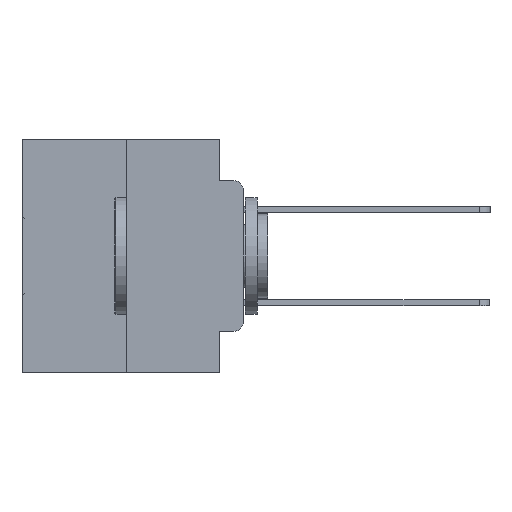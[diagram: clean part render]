
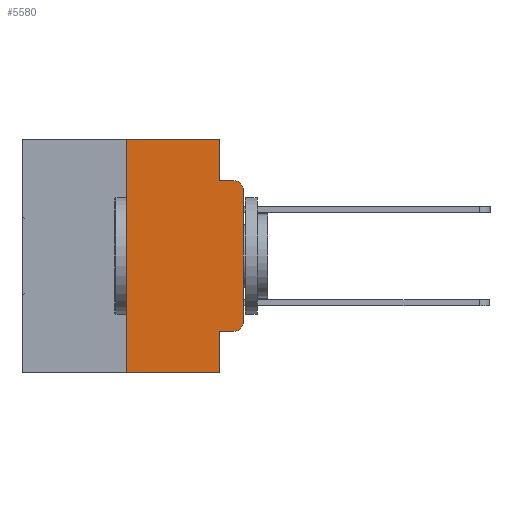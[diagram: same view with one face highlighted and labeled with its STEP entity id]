
A CAD part, left-side view. The second image highlights one B-rep face of the part: STEP entity #5580.
In plain terms, the highlighted planar face has unit normal (-1, 0, 0).
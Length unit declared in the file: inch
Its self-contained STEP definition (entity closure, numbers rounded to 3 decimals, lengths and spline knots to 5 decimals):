
#1508 = VERTEX_POINT ( 'NONE', #18379 ) ;
#1901 = AXIS2_PLACEMENT_3D ( 'NONE', #23226, #7736, #25802 ) ;
#2089 = CARTESIAN_POINT ( 'NONE',  ( 0., 0., -0.3915 ) ) ;
#2698 = CARTESIAN_POINT ( 'NONE',  ( 0., 0.051, 0. ) ) ;
#4531 = VECTOR ( 'NONE', #22962, 39.37008 ) ;
#4701 = EDGE_CURVE ( 'NONE', #5021, #1508, #15655, .T. ) ;
#5004 = AXIS2_PLACEMENT_3D ( 'NONE', #18978, #13904, #31989 ) ;
#5021 = VERTEX_POINT ( 'NONE', #19352 ) ;
#5310 = LINE ( 'NONE', #20338, #4531 ) ;
#5507 = LINE ( 'NONE', #14008, #32211 ) ;
#5580 = ADVANCED_FACE ( 'NONE', ( #9167 ), #13799, .F. ) ;
#6007 = EDGE_CURVE ( 'NONE', #32028, #27870, #29328, .T. ) ;
#6123 = VECTOR ( 'NONE', #23353, 39.37008 ) ;
#7227 = LINE ( 'NONE', #28027, #20176 ) ;
#7736 = DIRECTION ( 'NONE',  ( -1., 0., 0. ) ) ;
#7873 = EDGE_CURVE ( 'NONE', #24982, #12171, #5310, .T. ) ;
#7877 = DIRECTION ( 'NONE',  ( 0., 0., 1. ) ) ;
#8230 = ORIENTED_EDGE ( 'NONE', *, *, #7873, .T. ) ;
#8566 = EDGE_CURVE ( 'NONE', #12171, #15142, #11741, .T. ) ;
#9167 = FACE_OUTER_BOUND ( 'NONE', #31209, .T. ) ;
#9393 = EDGE_CURVE ( 'NONE', #18142, #24982, #27039, .T. ) ;
#10222 = ORIENTED_EDGE ( 'NONE', *, *, #30271, .F. ) ;
#10917 = VECTOR ( 'NONE', #22085, 39.37008 ) ;
#11630 = CARTESIAN_POINT ( 'NONE',  ( 0., 0.051, -0.4115 ) ) ;
#11741 = CIRCLE ( 'NONE', #28651, 0.02 ) ;
#12171 = VERTEX_POINT ( 'NONE', #19094 ) ;
#12544 = ORIENTED_EDGE ( 'NONE', *, *, #25397, .F. ) ;
#12953 = CARTESIAN_POINT ( 'NONE',  ( 0., 0.02, -0.1085 ) ) ;
#13072 = CARTESIAN_POINT ( 'NONE',  ( 0., 0.25, 0. ) ) ;
#13098 = ORIENTED_EDGE ( 'NONE', *, *, #4701, .F. ) ;
#13647 = EDGE_CURVE ( 'NONE', #31257, #23608, #20345, .T. ) ;
#13799 = PLANE ( 'NONE',  #5004 ) ;
#13904 = DIRECTION ( 'NONE',  ( 1., 0., 0. ) ) ;
#13960 = VECTOR ( 'NONE', #7877, 39.37008 ) ;
#14008 = CARTESIAN_POINT ( 'NONE',  ( 0., 0.051, -0.0885 ) ) ;
#14865 = CARTESIAN_POINT ( 'NONE',  ( 0., 0.25, -0.5 ) ) ;
#15142 = VERTEX_POINT ( 'NONE', #26522 ) ;
#15550 = DIRECTION ( 'NONE',  ( 0., 0., -1. ) ) ;
#15655 = LINE ( 'NONE', #2698, #21731 ) ;
#17257 = CARTESIAN_POINT ( 'NONE',  ( 0., 0.02, -0.4115 ) ) ;
#18133 = DIRECTION ( 'NONE',  ( 0., 0., -1. ) ) ;
#18142 = VERTEX_POINT ( 'NONE', #17257 ) ;
#18379 = CARTESIAN_POINT ( 'NONE',  ( 0., 0.051, -0.0885 ) ) ;
#18784 = ORIENTED_EDGE ( 'NONE', *, *, #13647, .F. ) ;
#18978 = CARTESIAN_POINT ( 'NONE',  ( 0., 0.473, 0. ) ) ;
#19094 = CARTESIAN_POINT ( 'NONE',  ( 0., 0., -0.1085 ) ) ;
#19352 = CARTESIAN_POINT ( 'NONE',  ( 0., 0.051, 0. ) ) ;
#19676 = ORIENTED_EDGE ( 'NONE', *, *, #24280, .T. ) ;
#19882 = LINE ( 'NONE', #20746, #6123 ) ;
#20176 = VECTOR ( 'NONE', #22985, 39.37008 ) ;
#20338 = CARTESIAN_POINT ( 'NONE',  ( 0., 0., 0. ) ) ;
#20345 = LINE ( 'NONE', #25717, #27195 ) ;
#20746 = CARTESIAN_POINT ( 'NONE',  ( 0., 0.051, -0.4115 ) ) ;
#21070 = ORIENTED_EDGE ( 'NONE', *, *, #6007, .F. ) ;
#21403 = ORIENTED_EDGE ( 'NONE', *, *, #8566, .T. ) ;
#21731 = VECTOR ( 'NONE', #18133, 39.37008 ) ;
#22085 = DIRECTION ( 'NONE',  ( 0., -1., 0. ) ) ;
#22962 = DIRECTION ( 'NONE',  ( 0., 0., 1. ) ) ;
#22985 = DIRECTION ( 'NONE',  ( 0., -1., 0. ) ) ;
#23226 = CARTESIAN_POINT ( 'NONE',  ( 0., 0.02, -0.3915 ) ) ;
#23353 = DIRECTION ( 'NONE',  ( 0., -1., 0. ) ) ;
#23608 = VERTEX_POINT ( 'NONE', #31699 ) ;
#24280 = EDGE_CURVE ( 'NONE', #32028, #23608, #25462, .T. ) ;
#24982 = VERTEX_POINT ( 'NONE', #2089 ) ;
#25273 = CARTESIAN_POINT ( 'NONE',  ( 0., 0.25, 0. ) ) ;
#25397 = EDGE_CURVE ( 'NONE', #1508, #15142, #5507, .T. ) ;
#25462 = LINE ( 'NONE', #29778, #10917 ) ;
#25717 = CARTESIAN_POINT ( 'NONE',  ( 0., 0.051, 0. ) ) ;
#25802 = DIRECTION ( 'NONE',  ( 0., 0., -1. ) ) ;
#26522 = CARTESIAN_POINT ( 'NONE',  ( 0., 0.02, -0.0885 ) ) ;
#27039 = CIRCLE ( 'NONE', #1901, 0.02 ) ;
#27195 = VECTOR ( 'NONE', #30938, 39.37008 ) ;
#27870 = VERTEX_POINT ( 'NONE', #25273 ) ;
#28027 = CARTESIAN_POINT ( 'NONE',  ( 0., 0.473, 0. ) ) ;
#28047 = EDGE_CURVE ( 'NONE', #31257, #18142, #19882, .T. ) ;
#28651 = AXIS2_PLACEMENT_3D ( 'NONE', #12953, #31040, #15550 ) ;
#29328 = LINE ( 'NONE', #13072, #13960 ) ;
#29778 = CARTESIAN_POINT ( 'NONE',  ( 0., 0.473, -0.5 ) ) ;
#30271 = EDGE_CURVE ( 'NONE', #27870, #5021, #7227, .T. ) ;
#30938 = DIRECTION ( 'NONE',  ( 0., 0., -1. ) ) ;
#31040 = DIRECTION ( 'NONE',  ( -1., 0., 0. ) ) ;
#31209 = EDGE_LOOP ( 'NONE', ( #8230, #21403, #12544, #13098, #10222, #21070, #19676, #18784, #32196, #32582 ) ) ;
#31257 = VERTEX_POINT ( 'NONE', #11630 ) ;
#31699 = CARTESIAN_POINT ( 'NONE',  ( 0., 0.051, -0.5 ) ) ;
#31989 = DIRECTION ( 'NONE',  ( 0., 0., -1. ) ) ;
#32028 = VERTEX_POINT ( 'NONE', #14865 ) ;
#32079 = DIRECTION ( 'NONE',  ( 0., -1., 0. ) ) ;
#32196 = ORIENTED_EDGE ( 'NONE', *, *, #28047, .T. ) ;
#32211 = VECTOR ( 'NONE', #32079, 39.37008 ) ;
#32582 = ORIENTED_EDGE ( 'NONE', *, *, #9393, .T. ) ;
